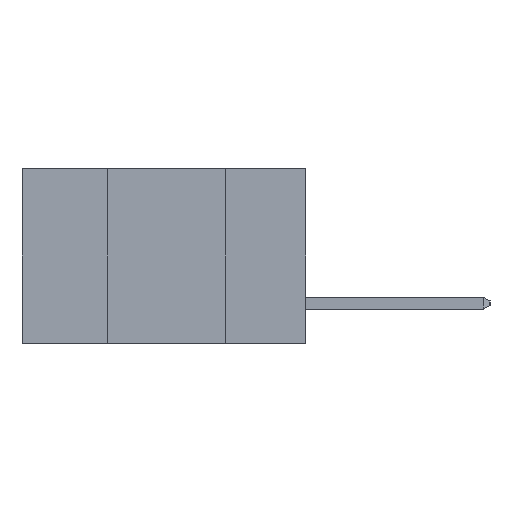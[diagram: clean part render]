
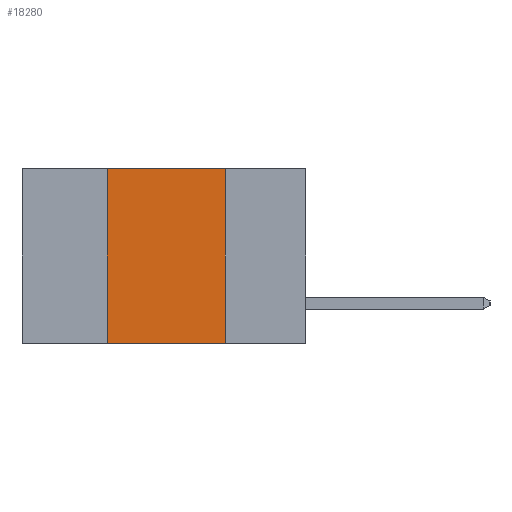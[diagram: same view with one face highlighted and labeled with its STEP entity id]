
A CAD part, left-side view. The second image highlights one B-rep face of the part: STEP entity #18280.
In plain terms, the highlighted planar face has unit normal (-1, 0, 0).
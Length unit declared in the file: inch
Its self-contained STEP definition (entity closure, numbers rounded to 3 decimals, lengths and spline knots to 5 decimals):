
#265 = ORIENTED_EDGE ( 'NONE', *, *, #17494, .F. ) ;
#1272 = AXIS2_PLACEMENT_3D ( 'NONE', #2181, #16393, #4262 ) ;
#1821 = VERTEX_POINT ( 'NONE', #5254 ) ;
#1854 = ORIENTED_EDGE ( 'NONE', *, *, #21679, .F. ) ;
#2181 = CARTESIAN_POINT ( 'NONE',  ( 0., 0.6, 0. ) ) ;
#3147 = VERTEX_POINT ( 'NONE', #19924 ) ;
#3605 = DIRECTION ( 'NONE',  ( 0., 0., 1. ) ) ;
#3641 = VERTEX_POINT ( 'NONE', #20205 ) ;
#3847 = CARTESIAN_POINT ( 'NONE',  ( 0., 0.6, 0. ) ) ;
#4262 = DIRECTION ( 'NONE',  ( 0., 0., -1. ) ) ;
#4301 = VECTOR ( 'NONE', #3605, 39.37008 ) ;
#4312 = VECTOR ( 'NONE', #21530, 39.37008 ) ;
#4979 = FACE_OUTER_BOUND ( 'NONE', #6123, .T. ) ;
#5254 = CARTESIAN_POINT ( 'NONE',  ( 0., 0.17, -0.37 ) ) ;
#5937 = DIRECTION ( 'NONE',  ( 0., -1., 0. ) ) ;
#6050 = CARTESIAN_POINT ( 'NONE',  ( 0., 0.42, 0. ) ) ;
#6123 = EDGE_LOOP ( 'NONE', ( #1854, #265, #14281, #12116 ) ) ;
#8816 = VERTEX_POINT ( 'NONE', #6050 ) ;
#10422 = LINE ( 'NONE', #19453, #4312 ) ;
#12116 = ORIENTED_EDGE ( 'NONE', *, *, #19587, .T. ) ;
#12241 = CARTESIAN_POINT ( 'NONE',  ( 0., 0.6, -0.37 ) ) ;
#12370 = PLANE ( 'NONE',  #1272 ) ;
#13257 = VECTOR ( 'NONE', #5937, 39.37008 ) ;
#14281 = ORIENTED_EDGE ( 'NONE', *, *, #19421, .F. ) ;
#16022 = LINE ( 'NONE', #12241, #21464 ) ;
#16393 = DIRECTION ( 'NONE',  ( 1., 0., 0. ) ) ;
#17494 = EDGE_CURVE ( 'NONE', #8816, #3641, #24115, .T. ) ;
#17765 = CARTESIAN_POINT ( 'NONE',  ( 0., 0.42, 0. ) ) ;
#18280 = ADVANCED_FACE ( 'NONE', ( #4979 ), #12370, .F. ) ;
#19421 = EDGE_CURVE ( 'NONE', #3147, #8816, #25336, .T. ) ;
#19453 = CARTESIAN_POINT ( 'NONE',  ( 0., 0.17, 0. ) ) ;
#19587 = EDGE_CURVE ( 'NONE', #3147, #1821, #16022, .T. ) ;
#19924 = CARTESIAN_POINT ( 'NONE',  ( 0., 0.42, -0.37 ) ) ;
#20205 = CARTESIAN_POINT ( 'NONE',  ( 0., 0.17, 0. ) ) ;
#21464 = VECTOR ( 'NONE', #24419, 39.37008 ) ;
#21530 = DIRECTION ( 'NONE',  ( 0., 0., -1. ) ) ;
#21679 = EDGE_CURVE ( 'NONE', #3641, #1821, #10422, .T. ) ;
#24115 = LINE ( 'NONE', #3847, #13257 ) ;
#24419 = DIRECTION ( 'NONE',  ( 0., -1., 0. ) ) ;
#25336 = LINE ( 'NONE', #17765, #4301 ) ;
